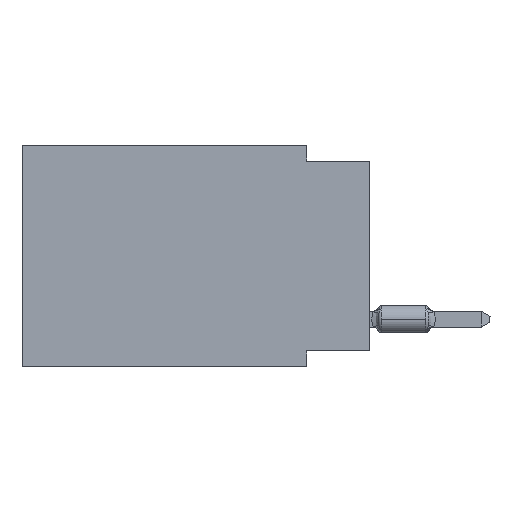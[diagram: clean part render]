
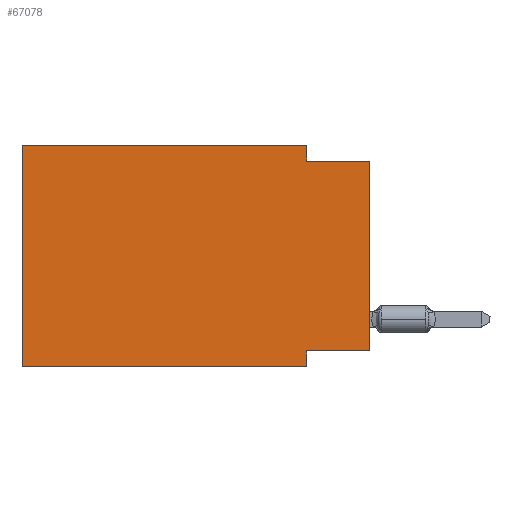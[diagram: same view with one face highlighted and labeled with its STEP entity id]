
A CAD part, left-side view. The second image highlights one B-rep face of the part: STEP entity #67078.
In plain terms, the highlighted planar face has unit normal (-1, 0, 0).
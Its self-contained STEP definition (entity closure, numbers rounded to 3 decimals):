
#201 = ORIENTED_EDGE ( 'NONE', *, *, #45421, .F. ) ;
#1231 = LINE ( 'NONE', #43416, #38657 ) ;
#3097 = VERTEX_POINT ( 'NONE', #14369 ) ;
#3688 = CARTESIAN_POINT ( 'NONE',  ( 0., 2.54, 0. ) ) ;
#5684 = CARTESIAN_POINT ( 'NONE',  ( 0., 0., 0. ) ) ;
#5745 = ORIENTED_EDGE ( 'NONE', *, *, #40826, .T. ) ;
#6485 = EDGE_CURVE ( 'NONE', #55787, #3097, #59296, .T. ) ;
#8605 = CARTESIAN_POINT ( 'NONE',  ( 0., 2.54, -8.89 ) ) ;
#8657 = VERTEX_POINT ( 'NONE', #14105 ) ;
#9935 = VECTOR ( 'NONE', #12891, 1000. ) ;
#10227 = EDGE_CURVE ( 'NONE', #57727, #8657, #24385, .T. ) ;
#10525 = ORIENTED_EDGE ( 'NONE', *, *, #10227, .F. ) ;
#11572 = CARTESIAN_POINT ( 'NONE',  ( 0., 13.97, -8.89 ) ) ;
#12427 = EDGE_CURVE ( 'NONE', #13597, #55787, #1231, .T. ) ;
#12891 = DIRECTION ( 'NONE',  ( 0., -1., 0. ) ) ;
#13135 = ORIENTED_EDGE ( 'NONE', *, *, #12427, .F. ) ;
#13170 = DIRECTION ( 'NONE',  ( 0., 0., -1. ) ) ;
#13202 = DIRECTION ( 'NONE',  ( 0., 0., -1. ) ) ;
#13597 = VERTEX_POINT ( 'NONE', #58557 ) ;
#14105 = CARTESIAN_POINT ( 'NONE',  ( 0., 2.54, -8.255 ) ) ;
#14369 = CARTESIAN_POINT ( 'NONE',  ( 0., 2.54, -0.635 ) ) ;
#14466 = ORIENTED_EDGE ( 'NONE', *, *, #40720, .T. ) ;
#15119 = AXIS2_PLACEMENT_3D ( 'NONE', #40255, #36225, #13170 ) ;
#17031 = VERTEX_POINT ( 'NONE', #42704 ) ;
#18681 = FACE_OUTER_BOUND ( 'NONE', #54771, .T. ) ;
#18891 = CARTESIAN_POINT ( 'NONE',  ( 0., 0., -8.255 ) ) ;
#21090 = LINE ( 'NONE', #43377, #55572 ) ;
#21881 = CARTESIAN_POINT ( 'NONE',  ( 0., 2.54, 0. ) ) ;
#22879 = VECTOR ( 'NONE', #45199, 1000. ) ;
#24385 = LINE ( 'NONE', #18891, #48967 ) ;
#31175 = ORIENTED_EDGE ( 'NONE', *, *, #59814, .F. ) ;
#34693 = VECTOR ( 'NONE', #64938, 1000. ) ;
#36225 = DIRECTION ( 'NONE',  ( 1., 0., 0. ) ) ;
#38657 = VECTOR ( 'NONE', #55150, 1000. ) ;
#40255 = CARTESIAN_POINT ( 'NONE',  ( 0., 13.97, 0. ) ) ;
#40720 = EDGE_CURVE ( 'NONE', #54672, #66404, #21090, .T. ) ;
#40826 = EDGE_CURVE ( 'NONE', #57727, #17031, #55820, .T. ) ;
#41970 = CARTESIAN_POINT ( 'NONE',  ( 0., 2.54, -8.89 ) ) ;
#42210 = CARTESIAN_POINT ( 'NONE',  ( 0., 0., -8.255 ) ) ;
#42704 = CARTESIAN_POINT ( 'NONE',  ( 0., 0., -0.635 ) ) ;
#43377 = CARTESIAN_POINT ( 'NONE',  ( 0., 13.97, -8.89 ) ) ;
#43416 = CARTESIAN_POINT ( 'NONE',  ( 0., 13.97, 0. ) ) ;
#45199 = DIRECTION ( 'NONE',  ( 0., 0., 1. ) ) ;
#45421 = EDGE_CURVE ( 'NONE', #8657, #66404, #71161, .T. ) ;
#48967 = VECTOR ( 'NONE', #67926, 1000. ) ;
#50352 = DIRECTION ( 'NONE',  ( 0., 0., 1. ) ) ;
#51077 = LINE ( 'NONE', #61681, #61356 ) ;
#54672 = VERTEX_POINT ( 'NONE', #11572 ) ;
#54771 = EDGE_LOOP ( 'NONE', ( #5745, #60453, #64035, #13135, #31175, #14466, #201, #10525 ) ) ;
#55150 = DIRECTION ( 'NONE',  ( 0., -1., 0. ) ) ;
#55572 = VECTOR ( 'NONE', #65702, 1000. ) ;
#55787 = VERTEX_POINT ( 'NONE', #21881 ) ;
#55820 = LINE ( 'NONE', #5684, #22879 ) ;
#57727 = VERTEX_POINT ( 'NONE', #42210 ) ;
#58557 = CARTESIAN_POINT ( 'NONE',  ( 0., 13.97, 0. ) ) ;
#58663 = EDGE_CURVE ( 'NONE', #3097, #17031, #68878, .T. ) ;
#59296 = LINE ( 'NONE', #3688, #70818 ) ;
#59814 = EDGE_CURVE ( 'NONE', #54672, #13597, #51077, .T. ) ;
#60453 = ORIENTED_EDGE ( 'NONE', *, *, #58663, .F. ) ;
#61356 = VECTOR ( 'NONE', #50352, 1000. ) ;
#61681 = CARTESIAN_POINT ( 'NONE',  ( 0., 13.97, 0. ) ) ;
#63046 = CARTESIAN_POINT ( 'NONE',  ( 0., 0., -0.635 ) ) ;
#63321 = PLANE ( 'NONE',  #15119 ) ;
#64035 = ORIENTED_EDGE ( 'NONE', *, *, #6485, .F. ) ;
#64938 = DIRECTION ( 'NONE',  ( 0., 0., -1. ) ) ;
#65702 = DIRECTION ( 'NONE',  ( 0., -1., 0. ) ) ;
#66404 = VERTEX_POINT ( 'NONE', #41970 ) ;
#67078 = ADVANCED_FACE ( 'NONE', ( #18681 ), #63321, .F. ) ;
#67926 = DIRECTION ( 'NONE',  ( 0., 1., 0. ) ) ;
#68878 = LINE ( 'NONE', #63046, #9935 ) ;
#70818 = VECTOR ( 'NONE', #13202, 1000. ) ;
#71161 = LINE ( 'NONE', #8605, #34693 ) ;
